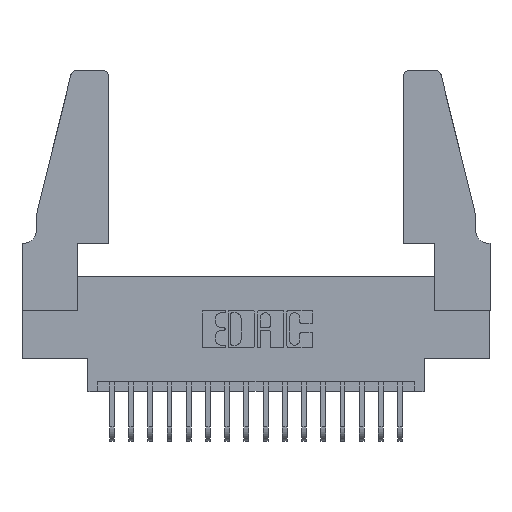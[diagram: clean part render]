
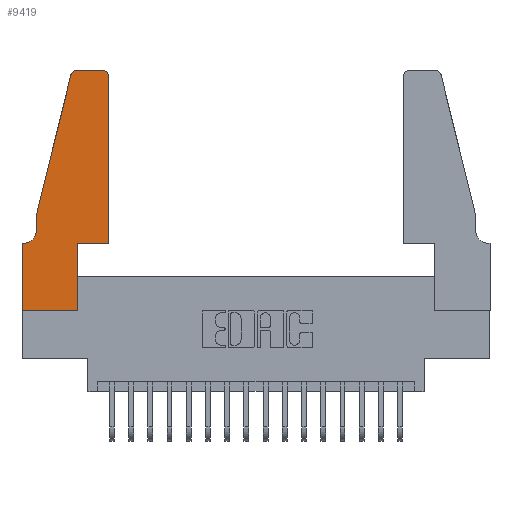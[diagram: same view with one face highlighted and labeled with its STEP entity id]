
A CAD part, top view. The second image highlights one B-rep face of the part: STEP entity #9419.
In plain terms, the highlighted planar face has unit normal (0, 0, 1).
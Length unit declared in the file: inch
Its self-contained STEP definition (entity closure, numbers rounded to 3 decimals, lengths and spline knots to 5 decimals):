
#65 = CARTESIAN_POINT ( 'NONE',  ( 0.284, 1.22, 0.37 ) ) ;
#184 = VERTEX_POINT ( 'NONE', #16309 ) ;
#437 = LINE ( 'NONE', #14905, #3785 ) ;
#508 = DIRECTION ( 'NONE',  ( -1., 0., 0. ) ) ;
#580 = CARTESIAN_POINT ( 'NONE',  ( 0.2865, 0., 0.37 ) ) ;
#945 = AXIS2_PLACEMENT_3D ( 'NONE', #12679, #4396, #14041 ) ;
#946 = VERTEX_POINT ( 'NONE', #10394 ) ;
#1458 = ORIENTED_EDGE ( 'NONE', *, *, #15788, .T. ) ;
#1470 = DIRECTION ( 'NONE',  ( 1., 0., 0. ) ) ;
#2395 = EDGE_CURVE ( 'NONE', #5156, #2879, #12889, .T. ) ;
#2440 = LINE ( 'NONE', #9189, #9448 ) ;
#2477 = LINE ( 'NONE', #15560, #6625 ) ;
#2532 = ORIENTED_EDGE ( 'NONE', *, *, #17606, .T. ) ;
#2879 = VERTEX_POINT ( 'NONE', #12972 ) ;
#3059 = CARTESIAN_POINT ( 'NONE',  ( 0.0755, 0.35, 0.37 ) ) ;
#3113 = DIRECTION ( 'NONE',  ( 1., 0., 0. ) ) ;
#3714 = VECTOR ( 'NONE', #3113, 39.37008 ) ;
#3785 = VECTOR ( 'NONE', #9492, 39.37008 ) ;
#3859 = DIRECTION ( 'NONE',  ( 0., 0., 1. ) ) ;
#3872 = DIRECTION ( 'NONE',  ( 0., -1., 0. ) ) ;
#4267 = EDGE_CURVE ( 'NONE', #184, #13213, #2440, .T. ) ;
#4396 = DIRECTION ( 'NONE',  ( 0., 0., -1. ) ) ;
#4527 = CARTESIAN_POINT ( 'NONE',  ( 0.0055, 0.35, 0.37 ) ) ;
#4856 = EDGE_CURVE ( 'NONE', #9564, #5156, #9094, .T. ) ;
#5085 = AXIS2_PLACEMENT_3D ( 'NONE', #5237, #6638, #16249 ) ;
#5156 = VERTEX_POINT ( 'NONE', #11391 ) ;
#5237 = CARTESIAN_POINT ( 'NONE',  ( 0., 0.35, 0.37 ) ) ;
#5811 = LINE ( 'NONE', #11388, #16774 ) ;
#5851 = DIRECTION ( 'NONE',  ( 0., -1., 0. ) ) ;
#6152 = LINE ( 'NONE', #3059, #9431 ) ;
#6405 = ORIENTED_EDGE ( 'NONE', *, *, #14697, .T. ) ;
#6453 = LINE ( 'NONE', #10378, #13778 ) ;
#6556 = ORIENTED_EDGE ( 'NONE', *, *, #8421, .T. ) ;
#6625 = VECTOR ( 'NONE', #7343, 39.37008 ) ;
#6638 = DIRECTION ( 'NONE',  ( 0., 0., 1. ) ) ;
#7142 = ORIENTED_EDGE ( 'NONE', *, *, #7178, .T. ) ;
#7178 = EDGE_CURVE ( 'NONE', #11810, #13958, #17110, .T. ) ;
#7292 = CARTESIAN_POINT ( 'NONE',  ( 0., 0., 0.37 ) ) ;
#7343 = DIRECTION ( 'NONE',  ( 0., 1., 0. ) ) ;
#7454 = ORIENTED_EDGE ( 'NONE', *, *, #4267, .T. ) ;
#7540 = AXIS2_PLACEMENT_3D ( 'NONE', #12172, #3859, #13506 ) ;
#7654 = EDGE_CURVE ( 'NONE', #2879, #184, #15823, .T. ) ;
#7657 = ORIENTED_EDGE ( 'NONE', *, *, #14539, .T. ) ;
#8421 = EDGE_CURVE ( 'NONE', #12551, #13446, #14702, .T. ) ;
#8562 = VERTEX_POINT ( 'NONE', #15818 ) ;
#8716 = LINE ( 'NONE', #9421, #15996 ) ;
#8783 = EDGE_CURVE ( 'NONE', #8562, #12551, #8716, .T. ) ;
#9094 = CIRCLE ( 'NONE', #7540, 0.03 ) ;
#9189 = CARTESIAN_POINT ( 'NONE',  ( 0.0755, 0.5, 0.37 ) ) ;
#9419 = ADVANCED_FACE ( 'NONE', ( #15318 ), #13498, .T. ) ;
#9421 = CARTESIAN_POINT ( 'NONE',  ( 0., 0., 0.37 ) ) ;
#9431 = VECTOR ( 'NONE', #14070, 39.37008 ) ;
#9448 = VECTOR ( 'NONE', #13228, 39.37008 ) ;
#9492 = DIRECTION ( 'NONE',  ( 0., 1., 0. ) ) ;
#9564 = VERTEX_POINT ( 'NONE', #15237 ) ;
#9877 = DIRECTION ( 'NONE',  ( 0., 0., 1. ) ) ;
#10014 = CARTESIAN_POINT ( 'NONE',  ( 0.0755, 0.42, 0.37 ) ) ;
#10059 = VERTEX_POINT ( 'NONE', #10787 ) ;
#10378 = CARTESIAN_POINT ( 'NONE',  ( 0.4505, 0.35, 0.37 ) ) ;
#10394 = CARTESIAN_POINT ( 'NONE',  ( 0.4505, 0.35, 0.37 ) ) ;
#10611 = CARTESIAN_POINT ( 'NONE',  ( 0., 0., 0.37 ) ) ;
#10787 = CARTESIAN_POINT ( 'NONE',  ( 0.2865, 0.35, 0.37 ) ) ;
#10865 = EDGE_CURVE ( 'NONE', #946, #9564, #437, .T. ) ;
#11388 = CARTESIAN_POINT ( 'NONE',  ( 0.0755, 0.5, 0.37 ) ) ;
#11391 = CARTESIAN_POINT ( 'NONE',  ( 0.4205, 1.25, 0.37 ) ) ;
#11810 = VERTEX_POINT ( 'NONE', #10014 ) ;
#12172 = CARTESIAN_POINT ( 'NONE',  ( 0.4205, 1.22, 0.37 ) ) ;
#12551 = VERTEX_POINT ( 'NONE', #10611 ) ;
#12596 = CARTESIAN_POINT ( 'NONE',  ( 0.0755, 0.5, 0.37 ) ) ;
#12679 = CARTESIAN_POINT ( 'NONE',  ( 0.0055, 0.42, 0.37 ) ) ;
#12889 = LINE ( 'NONE', #15755, #16524 ) ;
#12972 = CARTESIAN_POINT ( 'NONE',  ( 0.284, 1.25, 0.37 ) ) ;
#13213 = VERTEX_POINT ( 'NONE', #12596 ) ;
#13228 = DIRECTION ( 'NONE',  ( -0.239, -0.971, 0. ) ) ;
#13446 = VERTEX_POINT ( 'NONE', #580 ) ;
#13498 = PLANE ( 'NONE',  #5085 ) ;
#13506 = DIRECTION ( 'NONE',  ( 1., 0., 0. ) ) ;
#13591 = ORIENTED_EDGE ( 'NONE', *, *, #2395, .T. ) ;
#13778 = VECTOR ( 'NONE', #14326, 39.37008 ) ;
#13958 = VERTEX_POINT ( 'NONE', #4527 ) ;
#14041 = DIRECTION ( 'NONE',  ( -1., 0., 0. ) ) ;
#14070 = DIRECTION ( 'NONE',  ( -1., 0., 0. ) ) ;
#14077 = ORIENTED_EDGE ( 'NONE', *, *, #8783, .T. ) ;
#14108 = ORIENTED_EDGE ( 'NONE', *, *, #4856, .T. ) ;
#14326 = DIRECTION ( 'NONE',  ( 1., 0., 0. ) ) ;
#14539 = EDGE_CURVE ( 'NONE', #13213, #11810, #5811, .T. ) ;
#14697 = EDGE_CURVE ( 'NONE', #10059, #946, #6453, .T. ) ;
#14702 = LINE ( 'NONE', #7292, #3714 ) ;
#14905 = CARTESIAN_POINT ( 'NONE',  ( 0.4505, 0.35, 0.37 ) ) ;
#15012 = ORIENTED_EDGE ( 'NONE', *, *, #10865, .T. ) ;
#15017 = ORIENTED_EDGE ( 'NONE', *, *, #7654, .T. ) ;
#15237 = CARTESIAN_POINT ( 'NONE',  ( 0.4505, 1.22, 0.37 ) ) ;
#15318 = FACE_OUTER_BOUND ( 'NONE', #17873, .T. ) ;
#15560 = CARTESIAN_POINT ( 'NONE',  ( 0.2865, 0.35, 0.37 ) ) ;
#15755 = CARTESIAN_POINT ( 'NONE',  ( 0.2605, 1.25, 0.37 ) ) ;
#15788 = EDGE_CURVE ( 'NONE', #13446, #10059, #2477, .T. ) ;
#15818 = CARTESIAN_POINT ( 'NONE',  ( 0., 0.35, 0.37 ) ) ;
#15823 = CIRCLE ( 'NONE', #16403, 0.03 ) ;
#15996 = VECTOR ( 'NONE', #3872, 39.37008 ) ;
#16249 = DIRECTION ( 'NONE',  ( 1., 0., 0. ) ) ;
#16309 = CARTESIAN_POINT ( 'NONE',  ( 0.25487, 1.22718, 0.37 ) ) ;
#16403 = AXIS2_PLACEMENT_3D ( 'NONE', #65, #9877, #1470 ) ;
#16524 = VECTOR ( 'NONE', #508, 39.37008 ) ;
#16774 = VECTOR ( 'NONE', #5851, 39.37008 ) ;
#17110 = CIRCLE ( 'NONE', #945, 0.07 ) ;
#17606 = EDGE_CURVE ( 'NONE', #13958, #8562, #6152, .T. ) ;
#17873 = EDGE_LOOP ( 'NONE', ( #13591, #15017, #7454, #7657, #7142, #2532, #14077, #6556, #1458, #6405, #15012, #14108 ) ) ;
